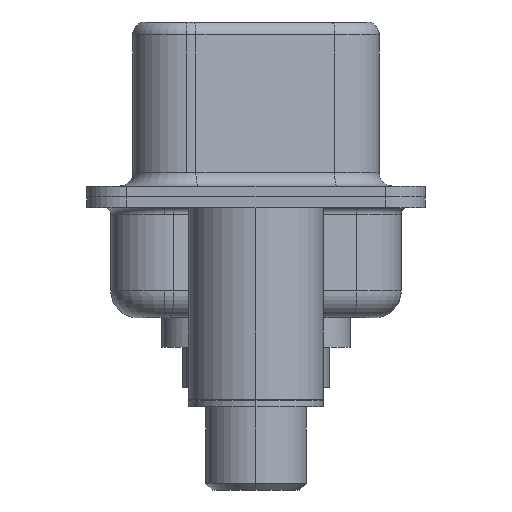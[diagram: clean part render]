
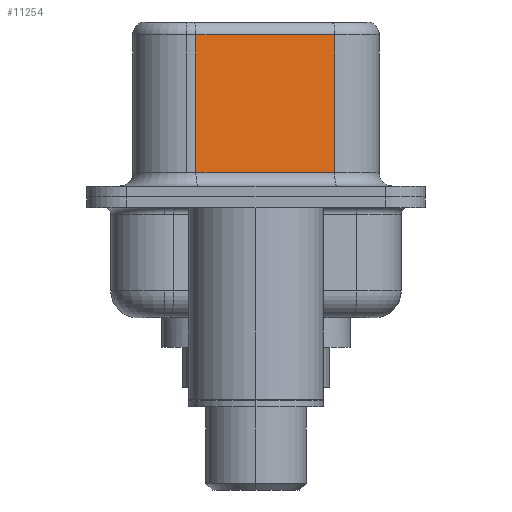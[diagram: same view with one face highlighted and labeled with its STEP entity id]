
A CAD part, left-side view. The second image highlights one B-rep face of the part: STEP entity #11254.
In plain terms, the highlighted planar face has unit normal (-0.985, -0.174, 0).
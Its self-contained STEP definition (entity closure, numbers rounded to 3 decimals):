
#124 = VERTEX_POINT ( 'NONE', #17521 ) ;
#187 = LINE ( 'NONE', #4833, #10831 ) ;
#1621 = ORIENTED_EDGE ( 'NONE', *, *, #15217, .F. ) ;
#1949 = DIRECTION ( 'NONE',  ( -0.174, 0.985, 0. ) ) ;
#2237 = ORIENTED_EDGE ( 'NONE', *, *, #12142, .T. ) ;
#2445 = CARTESIAN_POINT ( 'NONE',  ( 3.675, 2.233, 6.52 ) ) ;
#2856 = VERTEX_POINT ( 'NONE', #18518 ) ;
#2981 = VERTEX_POINT ( 'NONE', #8224 ) ;
#3896 = DIRECTION ( 'NONE',  ( 0., 0., -1. ) ) ;
#4833 = CARTESIAN_POINT ( 'NONE',  ( 4.585, -2.927, 6.02 ) ) ;
#6166 = DIRECTION ( 'NONE',  ( 0.174, -0.985, 0. ) ) ;
#6358 = PLANE ( 'NONE',  #15978 ) ;
#6943 = ORIENTED_EDGE ( 'NONE', *, *, #11213, .T. ) ;
#7171 = LINE ( 'NONE', #2445, #13957 ) ;
#8224 = CARTESIAN_POINT ( 'NONE',  ( 4.585, -2.927, 0.9 ) ) ;
#8698 = LINE ( 'NONE', #16099, #15878 ) ;
#9305 = DIRECTION ( 'NONE',  ( -0.174, 0.985, 0. ) ) ;
#9803 = VERTEX_POINT ( 'NONE', #13163 ) ;
#10493 = ORIENTED_EDGE ( 'NONE', *, *, #14005, .T. ) ;
#10746 = EDGE_LOOP ( 'NONE', ( #1621, #6943, #2237, #10493 ) ) ;
#10831 = VECTOR ( 'NONE', #1949, 1000. ) ;
#11213 = EDGE_CURVE ( 'NONE', #2856, #124, #187, .T. ) ;
#11254 = ADVANCED_FACE ( 'NONE', ( #17952 ), #6358, .F. ) ;
#12142 = EDGE_CURVE ( 'NONE', #124, #9803, #7171, .T. ) ;
#13163 = CARTESIAN_POINT ( 'NONE',  ( 3.675, 2.233, 0.9 ) ) ;
#13301 = DIRECTION ( 'NONE',  ( 0., 0., -1. ) ) ;
#13409 = CARTESIAN_POINT ( 'NONE',  ( 4.585, -2.927, 0.9 ) ) ;
#13957 = VECTOR ( 'NONE', #3896, 1000. ) ;
#14005 = EDGE_CURVE ( 'NONE', #9803, #2981, #16777, .T. ) ;
#15217 = EDGE_CURVE ( 'NONE', #2856, #2981, #8698, .T. ) ;
#15878 = VECTOR ( 'NONE', #13301, 1000. ) ;
#15978 = AXIS2_PLACEMENT_3D ( 'NONE', #16449, #17869, #9305 ) ;
#16099 = CARTESIAN_POINT ( 'NONE',  ( 4.585, -2.927, 6.52 ) ) ;
#16327 = VECTOR ( 'NONE', #6166, 1000. ) ;
#16449 = CARTESIAN_POINT ( 'NONE',  ( 4.585, -2.927, 6.52 ) ) ;
#16777 = LINE ( 'NONE', #13409, #16327 ) ;
#17521 = CARTESIAN_POINT ( 'NONE',  ( 3.675, 2.233, 6.02 ) ) ;
#17869 = DIRECTION ( 'NONE',  ( 0.985, 0.174, 0. ) ) ;
#17952 = FACE_OUTER_BOUND ( 'NONE', #10746, .T. ) ;
#18518 = CARTESIAN_POINT ( 'NONE',  ( 4.585, -2.927, 6.02 ) ) ;
